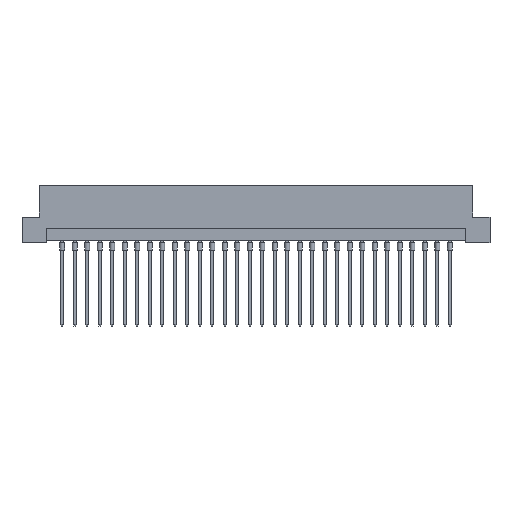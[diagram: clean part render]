
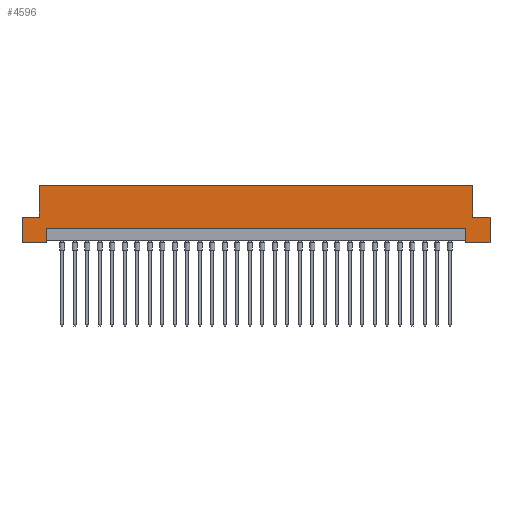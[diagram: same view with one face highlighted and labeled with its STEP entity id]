
A CAD part, front view. The second image highlights one B-rep face of the part: STEP entity #4596.
In plain terms, the highlighted planar face has unit normal (0, -1, 0).
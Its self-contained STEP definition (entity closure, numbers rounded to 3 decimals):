
#763 = CARTESIAN_POINT ( 'NONE',  ( -47.5, 0., 11.6 ) ) ;
#1090 = FACE_OUTER_BOUND ( 'NONE', #11742, .T. ) ;
#1192 = LINE ( 'NONE', #11434, #14470 ) ;
#1369 = CARTESIAN_POINT ( 'NONE',  ( -44., 0., 5.2 ) ) ;
#1606 = CARTESIAN_POINT ( 'NONE',  ( 44., 0., 5.2 ) ) ;
#1676 = LINE ( 'NONE', #5284, #6421 ) ;
#2034 = CARTESIAN_POINT ( 'NONE',  ( -47.5, 0., 11.6 ) ) ;
#2137 = VECTOR ( 'NONE', #2940, 1000. ) ;
#2149 = VERTEX_POINT ( 'NONE', #14044 ) ;
#2206 = DIRECTION ( 'NONE',  ( 0., 0., -1. ) ) ;
#2339 = VECTOR ( 'NONE', #6705, 1000. ) ;
#2936 = LINE ( 'NONE', #1606, #15993 ) ;
#2940 = DIRECTION ( 'NONE',  ( 1., 0., 0. ) ) ;
#3393 = LINE ( 'NONE', #8690, #11574 ) ;
#3410 = ORIENTED_EDGE ( 'NONE', *, *, #4147, .F. ) ;
#3424 = CARTESIAN_POINT ( 'NONE',  ( -42.6, 0., 0. ) ) ;
#3437 = PLANE ( 'NONE',  #4304 ) ;
#3454 = VERTEX_POINT ( 'NONE', #1369 ) ;
#3555 = ORIENTED_EDGE ( 'NONE', *, *, #9812, .T. ) ;
#3756 = EDGE_CURVE ( 'NONE', #15632, #10618, #3393, .T. ) ;
#3922 = EDGE_CURVE ( 'NONE', #6026, #7743, #14310, .T. ) ;
#4147 = EDGE_CURVE ( 'NONE', #9539, #5073, #7476, .T. ) ;
#4304 = AXIS2_PLACEMENT_3D ( 'NONE', #763, #13601, #13845 ) ;
#4470 = CARTESIAN_POINT ( 'NONE',  ( -47.5, 0., 5.2 ) ) ;
#4596 = ADVANCED_FACE ( 'NONE', ( #1090 ), #3437, .F. ) ;
#4869 = CARTESIAN_POINT ( 'NONE',  ( 47.5, 0., 0. ) ) ;
#5073 = VERTEX_POINT ( 'NONE', #5997 ) ;
#5284 = CARTESIAN_POINT ( 'NONE',  ( 42.6, 0., 2.9 ) ) ;
#5285 = ORIENTED_EDGE ( 'NONE', *, *, #9080, .F. ) ;
#5316 = CARTESIAN_POINT ( 'NONE',  ( -42.6, 0., 0.5 ) ) ;
#5363 = CARTESIAN_POINT ( 'NONE',  ( -47.5, 0., 0. ) ) ;
#5451 = EDGE_CURVE ( 'NONE', #9801, #2149, #1192, .T. ) ;
#5740 = ORIENTED_EDGE ( 'NONE', *, *, #3922, .F. ) ;
#5889 = VECTOR ( 'NONE', #13189, 1000. ) ;
#5935 = EDGE_CURVE ( 'NONE', #10618, #11421, #13848, .T. ) ;
#5997 = CARTESIAN_POINT ( 'NONE',  ( 44., 0., 11.6 ) ) ;
#6026 = VERTEX_POINT ( 'NONE', #15607 ) ;
#6399 = CARTESIAN_POINT ( 'NONE',  ( -47.5, 0., 0. ) ) ;
#6421 = VECTOR ( 'NONE', #12852, 1000. ) ;
#6630 = LINE ( 'NONE', #9315, #5889 ) ;
#6705 = DIRECTION ( 'NONE',  ( -1., 0., 0. ) ) ;
#7189 = EDGE_CURVE ( 'NONE', #8200, #3454, #8152, .T. ) ;
#7335 = CARTESIAN_POINT ( 'NONE',  ( -44., 0., 5.2 ) ) ;
#7476 = LINE ( 'NONE', #2034, #7798 ) ;
#7743 = VERTEX_POINT ( 'NONE', #3424 ) ;
#7798 = VECTOR ( 'NONE', #9840, 1000. ) ;
#8152 = LINE ( 'NONE', #9750, #2137 ) ;
#8200 = VERTEX_POINT ( 'NONE', #4470 ) ;
#8289 = ORIENTED_EDGE ( 'NONE', *, *, #5451, .T. ) ;
#8336 = CARTESIAN_POINT ( 'NONE',  ( -44., 0., 11.6 ) ) ;
#8482 = CARTESIAN_POINT ( 'NONE',  ( 47.5, 0., 0. ) ) ;
#8564 = CARTESIAN_POINT ( 'NONE',  ( -47.5, 0., 0. ) ) ;
#8633 = CARTESIAN_POINT ( 'NONE',  ( 47.5, 0., 5.2 ) ) ;
#8690 = CARTESIAN_POINT ( 'NONE',  ( 47.5, 0., 5.2 ) ) ;
#8701 = VERTEX_POINT ( 'NONE', #8564 ) ;
#9080 = EDGE_CURVE ( 'NONE', #3454, #9539, #16170, .T. ) ;
#9108 = DIRECTION ( 'NONE',  ( 0., 0., -1. ) ) ;
#9168 = VECTOR ( 'NONE', #14221, 1000. ) ;
#9211 = ORIENTED_EDGE ( 'NONE', *, *, #7189, .F. ) ;
#9315 = CARTESIAN_POINT ( 'NONE',  ( -47.5, 0., 0. ) ) ;
#9324 = CARTESIAN_POINT ( 'NONE',  ( 42.6, 0., 2.9 ) ) ;
#9539 = VERTEX_POINT ( 'NONE', #8336 ) ;
#9750 = CARTESIAN_POINT ( 'NONE',  ( -47.5, 0., 5.2 ) ) ;
#9801 = VERTEX_POINT ( 'NONE', #9324 ) ;
#9812 = EDGE_CURVE ( 'NONE', #15632, #5073, #2936, .T. ) ;
#9840 = DIRECTION ( 'NONE',  ( 1., 0., 0. ) ) ;
#10455 = VECTOR ( 'NONE', #13766, 1000. ) ;
#10618 = VERTEX_POINT ( 'NONE', #8633 ) ;
#10662 = CARTESIAN_POINT ( 'NONE',  ( 44., 0., 5.2 ) ) ;
#10932 = ORIENTED_EDGE ( 'NONE', *, *, #3756, .F. ) ;
#11047 = ORIENTED_EDGE ( 'NONE', *, *, #11599, .F. ) ;
#11421 = VERTEX_POINT ( 'NONE', #4869 ) ;
#11426 = ORIENTED_EDGE ( 'NONE', *, *, #5935, .F. ) ;
#11434 = CARTESIAN_POINT ( 'NONE',  ( 42.6, 0., 0.5 ) ) ;
#11533 = ORIENTED_EDGE ( 'NONE', *, *, #15025, .F. ) ;
#11563 = VECTOR ( 'NONE', #13645, 1000. ) ;
#11574 = VECTOR ( 'NONE', #14982, 1000. ) ;
#11582 = ORIENTED_EDGE ( 'NONE', *, *, #16241, .F. ) ;
#11599 = EDGE_CURVE ( 'NONE', #11421, #2149, #14351, .T. ) ;
#11742 = EDGE_LOOP ( 'NONE', ( #14546, #8289, #11047, #11426, #10932, #3555, #3410, #5285, #9211, #11582, #11533, #5740 ) ) ;
#12852 = DIRECTION ( 'NONE',  ( -1., 0., 0. ) ) ;
#13111 = DIRECTION ( 'NONE',  ( 0., 0., 1. ) ) ;
#13189 = DIRECTION ( 'NONE',  ( 0., 0., 1. ) ) ;
#13601 = DIRECTION ( 'NONE',  ( 0., 1., 0. ) ) ;
#13645 = DIRECTION ( 'NONE',  ( 0., 0., 1. ) ) ;
#13766 = DIRECTION ( 'NONE',  ( 0., 0., -1. ) ) ;
#13845 = DIRECTION ( 'NONE',  ( 0., 0., 1. ) ) ;
#13848 = LINE ( 'NONE', #8482, #10455 ) ;
#14044 = CARTESIAN_POINT ( 'NONE',  ( 42.6, 0., 0. ) ) ;
#14221 = DIRECTION ( 'NONE',  ( -1., 0., 0. ) ) ;
#14310 = LINE ( 'NONE', #5316, #14779 ) ;
#14351 = LINE ( 'NONE', #5363, #2339 ) ;
#14470 = VECTOR ( 'NONE', #2206, 1000. ) ;
#14546 = ORIENTED_EDGE ( 'NONE', *, *, #16223, .F. ) ;
#14779 = VECTOR ( 'NONE', #9108, 1000. ) ;
#14982 = DIRECTION ( 'NONE',  ( 1., 0., 0. ) ) ;
#15025 = EDGE_CURVE ( 'NONE', #7743, #8701, #15560, .T. ) ;
#15560 = LINE ( 'NONE', #6399, #9168 ) ;
#15607 = CARTESIAN_POINT ( 'NONE',  ( -42.6, 0., 2.9 ) ) ;
#15632 = VERTEX_POINT ( 'NONE', #10662 ) ;
#15993 = VECTOR ( 'NONE', #13111, 1000. ) ;
#16170 = LINE ( 'NONE', #7335, #11563 ) ;
#16223 = EDGE_CURVE ( 'NONE', #9801, #6026, #1676, .T. ) ;
#16241 = EDGE_CURVE ( 'NONE', #8701, #8200, #6630, .T. ) ;
